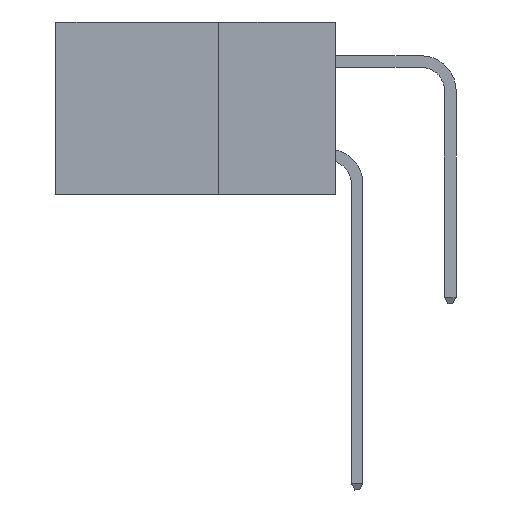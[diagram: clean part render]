
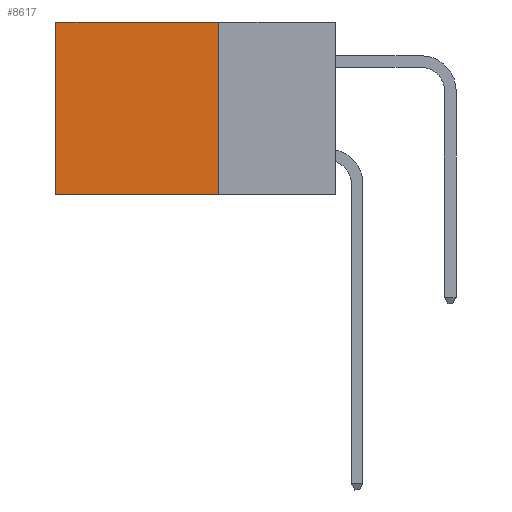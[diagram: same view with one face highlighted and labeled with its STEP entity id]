
A CAD part, left-side view. The second image highlights one B-rep face of the part: STEP entity #8617.
In plain terms, the highlighted planar face has unit normal (-1, 0, 0).
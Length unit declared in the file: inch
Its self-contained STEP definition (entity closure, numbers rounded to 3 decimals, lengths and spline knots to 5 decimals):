
#135 = VECTOR ( 'NONE', #8328, 39.37008 ) ;
#468 = VERTEX_POINT ( 'NONE', #4047 ) ;
#1241 = FACE_OUTER_BOUND ( 'NONE', #5525, .T. ) ;
#1699 = EDGE_CURVE ( 'NONE', #20306, #24614, #5565, .T. ) ;
#1852 = CARTESIAN_POINT ( 'NONE',  ( 0.2875, 0.25, -0.37 ) ) ;
#3525 = LINE ( 'NONE', #9189, #23060 ) ;
#4047 = CARTESIAN_POINT ( 'NONE',  ( 0.2875, 0.6, -0.37 ) ) ;
#5353 = DIRECTION ( 'NONE',  ( 0., 0., -1. ) ) ;
#5525 = EDGE_LOOP ( 'NONE', ( #14343, #8832, #6745, #15635 ) ) ;
#5565 = LINE ( 'NONE', #14515, #135 ) ;
#6745 = ORIENTED_EDGE ( 'NONE', *, *, #10974, .F. ) ;
#7170 = LINE ( 'NONE', #1852, #17033 ) ;
#7859 = PLANE ( 'NONE',  #9154 ) ;
#8056 = VERTEX_POINT ( 'NONE', #23255 ) ;
#8328 = DIRECTION ( 'NONE',  ( 0., 1., 0. ) ) ;
#8617 = ADVANCED_FACE ( 'NONE', ( #1241 ), #7859, .F. ) ;
#8832 = ORIENTED_EDGE ( 'NONE', *, *, #21133, .F. ) ;
#9154 = AXIS2_PLACEMENT_3D ( 'NONE', #21403, #9910, #23243 ) ;
#9189 = CARTESIAN_POINT ( 'NONE',  ( 0.2875, 0.6, 0. ) ) ;
#9910 = DIRECTION ( 'NONE',  ( 1., 0., 0. ) ) ;
#10697 = CARTESIAN_POINT ( 'NONE',  ( 0.2875, 0.6, 0. ) ) ;
#10974 = EDGE_CURVE ( 'NONE', #20306, #8056, #11421, .T. ) ;
#11194 = DIRECTION ( 'NONE',  ( 0., 0., -1. ) ) ;
#11291 = CARTESIAN_POINT ( 'NONE',  ( 0.2875, 0.25, 0. ) ) ;
#11421 = LINE ( 'NONE', #19107, #20976 ) ;
#14343 = ORIENTED_EDGE ( 'NONE', *, *, #15162, .T. ) ;
#14515 = CARTESIAN_POINT ( 'NONE',  ( 0.2875, 0.25, 0. ) ) ;
#15162 = EDGE_CURVE ( 'NONE', #24614, #468, #3525, .T. ) ;
#15635 = ORIENTED_EDGE ( 'NONE', *, *, #1699, .T. ) ;
#17033 = VECTOR ( 'NONE', #17761, 39.37008 ) ;
#17761 = DIRECTION ( 'NONE',  ( 0., 1., 0. ) ) ;
#19107 = CARTESIAN_POINT ( 'NONE',  ( 0.2875, 0.25, 0. ) ) ;
#20306 = VERTEX_POINT ( 'NONE', #11291 ) ;
#20976 = VECTOR ( 'NONE', #5353, 39.37008 ) ;
#21133 = EDGE_CURVE ( 'NONE', #8056, #468, #7170, .T. ) ;
#21403 = CARTESIAN_POINT ( 'NONE',  ( 0.2875, 0.25, 0. ) ) ;
#23060 = VECTOR ( 'NONE', #11194, 39.37008 ) ;
#23243 = DIRECTION ( 'NONE',  ( 0., 0., -1. ) ) ;
#23255 = CARTESIAN_POINT ( 'NONE',  ( 0.2875, 0.25, -0.37 ) ) ;
#24614 = VERTEX_POINT ( 'NONE', #10697 ) ;
